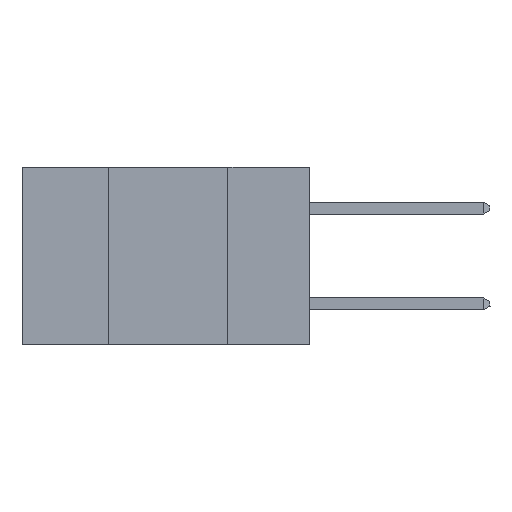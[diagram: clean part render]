
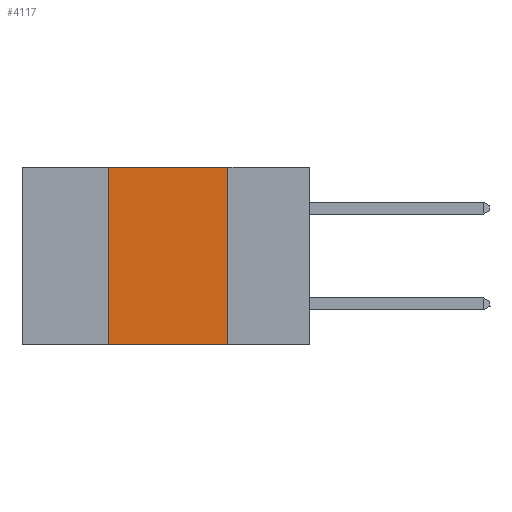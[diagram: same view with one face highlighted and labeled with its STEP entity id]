
A CAD part, left-side view. The second image highlights one B-rep face of the part: STEP entity #4117.
In plain terms, the highlighted planar face has unit normal (-1, 0, 0).
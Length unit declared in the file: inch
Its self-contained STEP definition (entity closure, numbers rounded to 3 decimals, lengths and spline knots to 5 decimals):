
#32 = CARTESIAN_POINT ( 'NONE',  ( 0., 0.17, -0.37 ) ) ;
#719 = CARTESIAN_POINT ( 'NONE',  ( 0., 0.6, 0. ) ) ;
#2237 = EDGE_CURVE ( 'NONE', #4448, #12746, #4474, .T. ) ;
#3186 = ORIENTED_EDGE ( 'NONE', *, *, #8568, .F. ) ;
#3277 = PLANE ( 'NONE',  #18417 ) ;
#3381 = VERTEX_POINT ( 'NONE', #9435 ) ;
#4117 = ADVANCED_FACE ( 'NONE', ( #19344 ), #3277, .F. ) ;
#4311 = DIRECTION ( 'NONE',  ( 0., 0., -1. ) ) ;
#4448 = VERTEX_POINT ( 'NONE', #8540 ) ;
#4474 = LINE ( 'NONE', #15601, #17408 ) ;
#4719 = VECTOR ( 'NONE', #11504, 39.37008 ) ;
#6097 = DIRECTION ( 'NONE',  ( 0., -1., 0. ) ) ;
#6202 = VECTOR ( 'NONE', #6097, 39.37008 ) ;
#6407 = EDGE_LOOP ( 'NONE', ( #21256, #3186, #15597, #17175 ) ) ;
#8528 = CARTESIAN_POINT ( 'NONE',  ( 0., 0.42, 0. ) ) ;
#8540 = CARTESIAN_POINT ( 'NONE',  ( 0., 0.42, -0.37 ) ) ;
#8568 = EDGE_CURVE ( 'NONE', #12746, #3381, #13139, .T. ) ;
#9435 = CARTESIAN_POINT ( 'NONE',  ( 0., 0.17, 0. ) ) ;
#9624 = LINE ( 'NONE', #15009, #4719 ) ;
#10430 = DIRECTION ( 'NONE',  ( 0., 0., -1. ) ) ;
#11504 = DIRECTION ( 'NONE',  ( 0., -1., 0. ) ) ;
#11679 = EDGE_CURVE ( 'NONE', #3381, #16434, #16734, .T. ) ;
#12746 = VERTEX_POINT ( 'NONE', #8528 ) ;
#13117 = CARTESIAN_POINT ( 'NONE',  ( 0., 0.17, 0. ) ) ;
#13139 = LINE ( 'NONE', #719, #6202 ) ;
#14165 = DIRECTION ( 'NONE',  ( 1., 0., 0. ) ) ;
#15009 = CARTESIAN_POINT ( 'NONE',  ( 0., 0.6, -0.37 ) ) ;
#15597 = ORIENTED_EDGE ( 'NONE', *, *, #2237, .F. ) ;
#15601 = CARTESIAN_POINT ( 'NONE',  ( 0., 0.42, 0. ) ) ;
#16434 = VERTEX_POINT ( 'NONE', #32 ) ;
#16734 = LINE ( 'NONE', #13117, #18998 ) ;
#17175 = ORIENTED_EDGE ( 'NONE', *, *, #19258, .T. ) ;
#17408 = VECTOR ( 'NONE', #22759, 39.37008 ) ;
#17796 = CARTESIAN_POINT ( 'NONE',  ( 0., 0.6, 0. ) ) ;
#18417 = AXIS2_PLACEMENT_3D ( 'NONE', #17796, #14165, #10430 ) ;
#18998 = VECTOR ( 'NONE', #4311, 39.37008 ) ;
#19258 = EDGE_CURVE ( 'NONE', #4448, #16434, #9624, .T. ) ;
#19344 = FACE_OUTER_BOUND ( 'NONE', #6407, .T. ) ;
#21256 = ORIENTED_EDGE ( 'NONE', *, *, #11679, .F. ) ;
#22759 = DIRECTION ( 'NONE',  ( 0., 0., 1. ) ) ;
